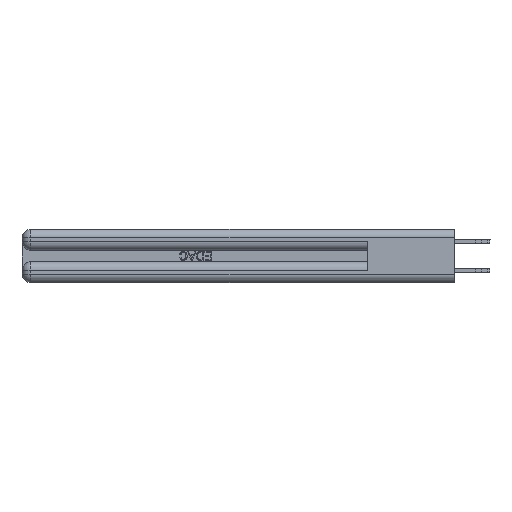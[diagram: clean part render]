
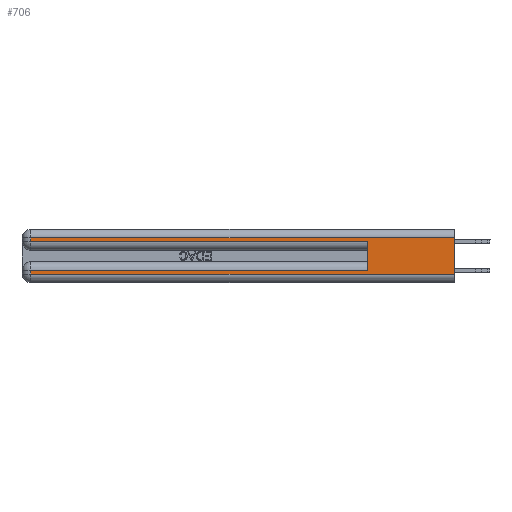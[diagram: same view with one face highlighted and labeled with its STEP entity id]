
A CAD part, left-side view. The second image highlights one B-rep face of the part: STEP entity #706.
In plain terms, the highlighted planar face has unit normal (-1, 0, 0).
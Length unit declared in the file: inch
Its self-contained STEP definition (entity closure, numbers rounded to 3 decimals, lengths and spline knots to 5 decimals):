
#49 = CARTESIAN_POINT ( 'NONE',  ( 0., 2.94, 0.285 ) ) ;
#397 = DIRECTION ( 'NONE',  ( 0., 0., -1. ) ) ;
#706 = ADVANCED_FACE ( 'NONE', ( #20234 ), #7400, .F. ) ;
#2336 = DIRECTION ( 'NONE',  ( 0., -1., 0. ) ) ;
#2369 = VERTEX_POINT ( 'NONE', #37230 ) ;
#3305 = CARTESIAN_POINT ( 'NONE',  ( 0., 0., 0.085 ) ) ;
#3421 = CARTESIAN_POINT ( 'NONE',  ( 0., 0.6, 0.285 ) ) ;
#3423 = VECTOR ( 'NONE', #16524, 39.37008 ) ;
#4031 = ORIENTED_EDGE ( 'NONE', *, *, #41788, .T. ) ;
#6012 = VERTEX_POINT ( 'NONE', #3421 ) ;
#6190 = ORIENTED_EDGE ( 'NONE', *, *, #38755, .T. ) ;
#6202 = VERTEX_POINT ( 'NONE', #17491 ) ;
#6940 = EDGE_LOOP ( 'NONE', ( #10327, #22250, #4031, #6190, #41200, #25329, #28882, #16450 ) ) ;
#7400 = PLANE ( 'NONE',  #28601 ) ;
#7523 = VECTOR ( 'NONE', #11087, 39.37008 ) ;
#7594 = VECTOR ( 'NONE', #22214, 39.37008 ) ;
#7814 = CARTESIAN_POINT ( 'NONE',  ( 0., 2.94, 0.085 ) ) ;
#7816 = CARTESIAN_POINT ( 'NONE',  ( 0., 0., 0.37 ) ) ;
#8179 = LINE ( 'NONE', #11422, #39604 ) ;
#8404 = VERTEX_POINT ( 'NONE', #27787 ) ;
#8997 = DIRECTION ( 'NONE',  ( 0., 0., 1. ) ) ;
#9853 = DIRECTION ( 'NONE',  ( 0., 1., 0. ) ) ;
#10264 = CARTESIAN_POINT ( 'NONE',  ( 0., 0., 0.06 ) ) ;
#10327 = ORIENTED_EDGE ( 'NONE', *, *, #24854, .F. ) ;
#11064 = LINE ( 'NONE', #22891, #3423 ) ;
#11087 = DIRECTION ( 'NONE',  ( 0., 0., -1. ) ) ;
#11422 = CARTESIAN_POINT ( 'NONE',  ( 0., 0.6, 0.145 ) ) ;
#13502 = LINE ( 'NONE', #3305, #18033 ) ;
#15801 = VERTEX_POINT ( 'NONE', #7814 ) ;
#16450 = ORIENTED_EDGE ( 'NONE', *, *, #34412, .T. ) ;
#16524 = DIRECTION ( 'NONE',  ( 0., 1., 0. ) ) ;
#17491 = CARTESIAN_POINT ( 'NONE',  ( 0., 0., 0.31 ) ) ;
#17982 = VECTOR ( 'NONE', #2336, 39.37008 ) ;
#18033 = VECTOR ( 'NONE', #9853, 39.37008 ) ;
#19344 = EDGE_CURVE ( 'NONE', #6202, #22761, #11064, .T. ) ;
#20234 = FACE_OUTER_BOUND ( 'NONE', #6940, .T. ) ;
#21179 = DIRECTION ( 'NONE',  ( 0., 0., -1. ) ) ;
#21635 = CARTESIAN_POINT ( 'NONE',  ( 0., 0., 0.285 ) ) ;
#22214 = DIRECTION ( 'NONE',  ( 0., -1., 0. ) ) ;
#22250 = ORIENTED_EDGE ( 'NONE', *, *, #19344, .T. ) ;
#22761 = VERTEX_POINT ( 'NONE', #39561 ) ;
#22891 = CARTESIAN_POINT ( 'NONE',  ( 0., 0., 0.31 ) ) ;
#23779 = LINE ( 'NONE', #7816, #7523 ) ;
#24164 = CARTESIAN_POINT ( 'NONE',  ( 0., 2.94, 0.37 ) ) ;
#24854 = EDGE_CURVE ( 'NONE', #6202, #36666, #23779, .T. ) ;
#25329 = ORIENTED_EDGE ( 'NONE', *, *, #41427, .T. ) ;
#26571 = LINE ( 'NONE', #21635, #17982 ) ;
#27787 = CARTESIAN_POINT ( 'NONE',  ( 0., 2.94, 0.06 ) ) ;
#28090 = VECTOR ( 'NONE', #21179, 39.37008 ) ;
#28601 = AXIS2_PLACEMENT_3D ( 'NONE', #30068, #30479, #34189 ) ;
#28882 = ORIENTED_EDGE ( 'NONE', *, *, #34174, .T. ) ;
#29654 = LINE ( 'NONE', #24164, #28090 ) ;
#30068 = CARTESIAN_POINT ( 'NONE',  ( 0., 0., 0.37 ) ) ;
#30479 = DIRECTION ( 'NONE',  ( 1., 0., 0. ) ) ;
#33199 = EDGE_CURVE ( 'NONE', #2369, #6012, #8179, .T. ) ;
#33276 = CARTESIAN_POINT ( 'NONE',  ( 0., 2.94, 0.37 ) ) ;
#34174 = EDGE_CURVE ( 'NONE', #15801, #8404, #40752, .T. ) ;
#34189 = DIRECTION ( 'NONE',  ( 0., 0., -1. ) ) ;
#34412 = EDGE_CURVE ( 'NONE', #8404, #36666, #41597, .T. ) ;
#36666 = VERTEX_POINT ( 'NONE', #10264 ) ;
#37230 = CARTESIAN_POINT ( 'NONE',  ( 0., 0.6, 0.085 ) ) ;
#38502 = CARTESIAN_POINT ( 'NONE',  ( 0., 0., 0.06 ) ) ;
#38755 = EDGE_CURVE ( 'NONE', #41395, #6012, #26571, .T. ) ;
#39561 = CARTESIAN_POINT ( 'NONE',  ( 0., 2.94, 0.31 ) ) ;
#39604 = VECTOR ( 'NONE', #8997, 39.37008 ) ;
#40752 = LINE ( 'NONE', #33276, #41223 ) ;
#41200 = ORIENTED_EDGE ( 'NONE', *, *, #33199, .F. ) ;
#41223 = VECTOR ( 'NONE', #397, 39.37008 ) ;
#41395 = VERTEX_POINT ( 'NONE', #49 ) ;
#41427 = EDGE_CURVE ( 'NONE', #2369, #15801, #13502, .T. ) ;
#41597 = LINE ( 'NONE', #38502, #7594 ) ;
#41788 = EDGE_CURVE ( 'NONE', #22761, #41395, #29654, .T. ) ;
